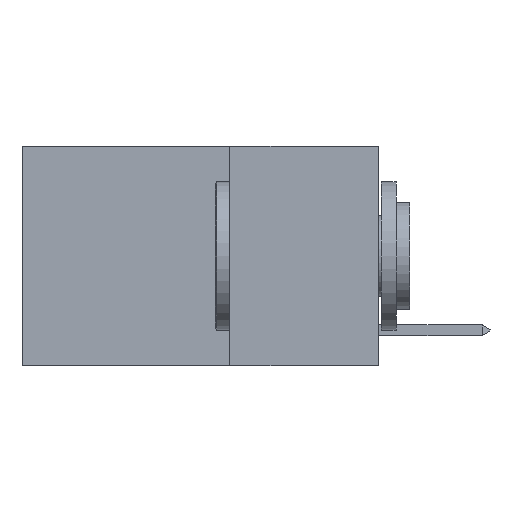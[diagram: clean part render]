
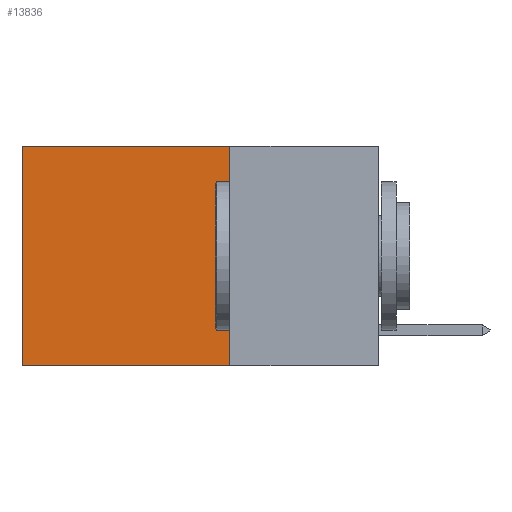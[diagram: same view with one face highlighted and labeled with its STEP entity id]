
A CAD part, left-side view. The second image highlights one B-rep face of the part: STEP entity #13836.
In plain terms, the highlighted planar face has unit normal (-1, 0, 0).
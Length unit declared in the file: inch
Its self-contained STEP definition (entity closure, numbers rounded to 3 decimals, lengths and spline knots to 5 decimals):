
#135 = DIRECTION ( 'NONE',  ( 1., 0., 0. ) ) ;
#320 = EDGE_CURVE ( 'NONE', #3753, #2390, #360, .T. ) ;
#360 = LINE ( 'NONE', #15862, #13298 ) ;
#1105 = CARTESIAN_POINT ( 'NONE',  ( 0.2625, 0.25, 0. ) ) ;
#1436 = LINE ( 'NONE', #1105, #14242 ) ;
#2034 = DIRECTION ( 'NONE',  ( 0., 0., -1. ) ) ;
#2390 = VERTEX_POINT ( 'NONE', #12998 ) ;
#2447 = DIRECTION ( 'NONE',  ( 0., 1., 0. ) ) ;
#3336 = CARTESIAN_POINT ( 'NONE',  ( 0.2625, 0.25, 0. ) ) ;
#3409 = CARTESIAN_POINT ( 'NONE',  ( 0.2625, 0.6, 0. ) ) ;
#3706 = CARTESIAN_POINT ( 'NONE',  ( 0.2625, 0.25, -0.37 ) ) ;
#3753 = VERTEX_POINT ( 'NONE', #3409 ) ;
#4026 = CARTESIAN_POINT ( 'NONE',  ( 0.2625, 0.25, 0. ) ) ;
#4997 = DIRECTION ( 'NONE',  ( 0., 1., 0. ) ) ;
#5090 = CARTESIAN_POINT ( 'NONE',  ( 0.2625, 0.25, -0.37 ) ) ;
#5809 = VERTEX_POINT ( 'NONE', #4026 ) ;
#6087 = FACE_OUTER_BOUND ( 'NONE', #13973, .T. ) ;
#6424 = ORIENTED_EDGE ( 'NONE', *, *, #10968, .F. ) ;
#6623 = PLANE ( 'NONE',  #14841 ) ;
#8691 = LINE ( 'NONE', #3706, #9075 ) ;
#9075 = VECTOR ( 'NONE', #4997, 39.37008 ) ;
#9098 = DIRECTION ( 'NONE',  ( 0., 0., -1. ) ) ;
#9346 = ORIENTED_EDGE ( 'NONE', *, *, #11131, .T. ) ;
#9860 = EDGE_CURVE ( 'NONE', #13188, #2390, #8691, .T. ) ;
#10968 = EDGE_CURVE ( 'NONE', #5809, #13188, #11267, .T. ) ;
#11131 = EDGE_CURVE ( 'NONE', #5809, #3753, #1436, .T. ) ;
#11267 = LINE ( 'NONE', #3336, #13731 ) ;
#12998 = CARTESIAN_POINT ( 'NONE',  ( 0.2625, 0.6, -0.37 ) ) ;
#13188 = VERTEX_POINT ( 'NONE', #5090 ) ;
#13233 = ORIENTED_EDGE ( 'NONE', *, *, #320, .T. ) ;
#13298 = VECTOR ( 'NONE', #16085, 39.37008 ) ;
#13731 = VECTOR ( 'NONE', #2034, 39.37008 ) ;
#13836 = ADVANCED_FACE ( 'NONE', ( #6087 ), #6623, .F. ) ;
#13973 = EDGE_LOOP ( 'NONE', ( #13233, #14934, #6424, #9346 ) ) ;
#14242 = VECTOR ( 'NONE', #2447, 39.37008 ) ;
#14841 = AXIS2_PLACEMENT_3D ( 'NONE', #15067, #135, #9098 ) ;
#14934 = ORIENTED_EDGE ( 'NONE', *, *, #9860, .F. ) ;
#15067 = CARTESIAN_POINT ( 'NONE',  ( 0.2625, 0.25, 0. ) ) ;
#15862 = CARTESIAN_POINT ( 'NONE',  ( 0.2625, 0.6, 0. ) ) ;
#16085 = DIRECTION ( 'NONE',  ( 0., 0., -1. ) ) ;
